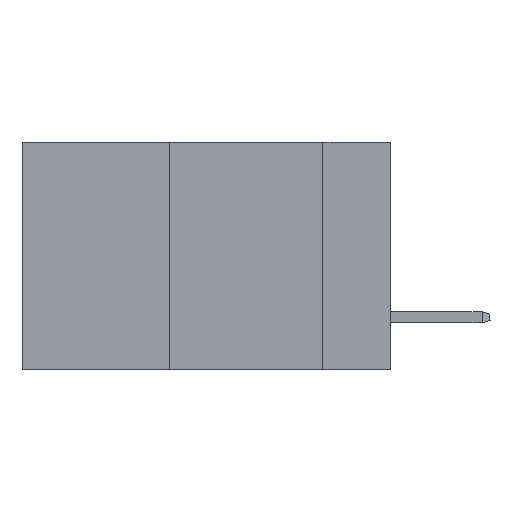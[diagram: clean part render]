
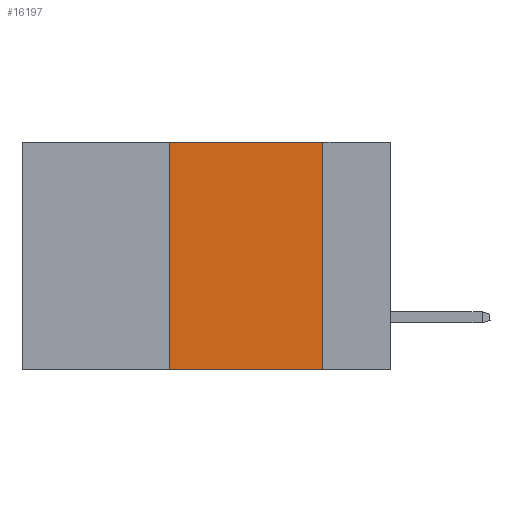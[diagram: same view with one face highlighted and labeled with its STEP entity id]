
A CAD part, left-side view. The second image highlights one B-rep face of the part: STEP entity #16197.
In plain terms, the highlighted planar face has unit normal (-1, 0, 0).
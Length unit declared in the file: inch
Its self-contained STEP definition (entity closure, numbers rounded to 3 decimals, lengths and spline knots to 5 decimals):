
#216 = EDGE_CURVE ( 'NONE', #1109, #6881, #2220, .T. ) ;
#749 = AXIS2_PLACEMENT_3D ( 'NONE', #18745, #6471, #18807 ) ;
#919 = VECTOR ( 'NONE', #16514, 39.37008 ) ;
#1109 = VERTEX_POINT ( 'NONE', #2105 ) ;
#1139 = DIRECTION ( 'NONE',  ( 0., -1., 0. ) ) ;
#1861 = LINE ( 'NONE', #10173, #919 ) ;
#2105 = CARTESIAN_POINT ( 'NONE',  ( 0., 0.36, 0. ) ) ;
#2220 = LINE ( 'NONE', #12105, #3463 ) ;
#2533 = VERTEX_POINT ( 'NONE', #7565 ) ;
#3463 = VECTOR ( 'NONE', #1139, 39.37008 ) ;
#4272 = FACE_OUTER_BOUND ( 'NONE', #13627, .T. ) ;
#4462 = DIRECTION ( 'NONE',  ( 0., -1., 0. ) ) ;
#6008 = CARTESIAN_POINT ( 'NONE',  ( 0., 0.11, 0. ) ) ;
#6471 = DIRECTION ( 'NONE',  ( 1., 0., 0. ) ) ;
#6881 = VERTEX_POINT ( 'NONE', #19606 ) ;
#7565 = CARTESIAN_POINT ( 'NONE',  ( 0., 0.11, -0.37 ) ) ;
#8038 = LINE ( 'NONE', #18457, #18959 ) ;
#8744 = ORIENTED_EDGE ( 'NONE', *, *, #14170, .F. ) ;
#10173 = CARTESIAN_POINT ( 'NONE',  ( 0., 0.36, 0. ) ) ;
#10858 = PLANE ( 'NONE',  #749 ) ;
#12105 = CARTESIAN_POINT ( 'NONE',  ( 0., 0.6, 0. ) ) ;
#12544 = VERTEX_POINT ( 'NONE', #14425 ) ;
#12859 = EDGE_CURVE ( 'NONE', #12544, #2533, #8038, .T. ) ;
#13627 = EDGE_LOOP ( 'NONE', ( #8744, #19149, #18332, #14003 ) ) ;
#14003 = ORIENTED_EDGE ( 'NONE', *, *, #12859, .T. ) ;
#14170 = EDGE_CURVE ( 'NONE', #6881, #2533, #15731, .T. ) ;
#14425 = CARTESIAN_POINT ( 'NONE',  ( 0., 0.36, -0.37 ) ) ;
#15369 = DIRECTION ( 'NONE',  ( 0., 0., -1. ) ) ;
#15731 = LINE ( 'NONE', #6008, #19145 ) ;
#16197 = ADVANCED_FACE ( 'NONE', ( #4272 ), #10858, .F. ) ;
#16514 = DIRECTION ( 'NONE',  ( 0., 0., 1. ) ) ;
#18132 = EDGE_CURVE ( 'NONE', #12544, #1109, #1861, .T. ) ;
#18332 = ORIENTED_EDGE ( 'NONE', *, *, #18132, .F. ) ;
#18457 = CARTESIAN_POINT ( 'NONE',  ( 0., 0.6, -0.37 ) ) ;
#18745 = CARTESIAN_POINT ( 'NONE',  ( 0., 0.6, 0. ) ) ;
#18807 = DIRECTION ( 'NONE',  ( 0., 0., -1. ) ) ;
#18959 = VECTOR ( 'NONE', #4462, 39.37008 ) ;
#19145 = VECTOR ( 'NONE', #15369, 39.37008 ) ;
#19149 = ORIENTED_EDGE ( 'NONE', *, *, #216, .F. ) ;
#19606 = CARTESIAN_POINT ( 'NONE',  ( 0., 0.11, 0. ) ) ;
